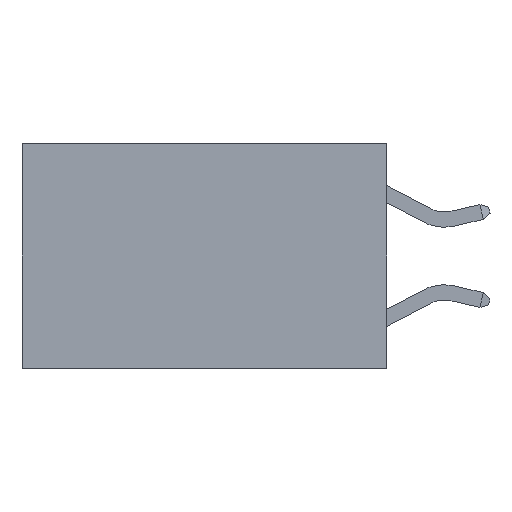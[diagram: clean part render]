
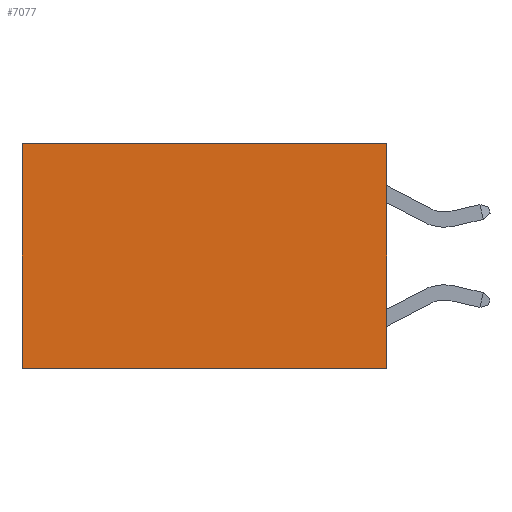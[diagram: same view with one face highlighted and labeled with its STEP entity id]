
A CAD part, left-side view. The second image highlights one B-rep face of the part: STEP entity #7077.
In plain terms, the highlighted planar face has unit normal (-1, 0, 0).
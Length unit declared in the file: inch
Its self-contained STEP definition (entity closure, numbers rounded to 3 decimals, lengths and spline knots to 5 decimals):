
#49 = DIRECTION ( 'NONE',  ( 1., 0., 0. ) ) ;
#55 = DIRECTION ( 'NONE',  ( 0., 1., 0. ) ) ;
#321 = VERTEX_POINT ( 'NONE', #4754 ) ;
#524 = VECTOR ( 'NONE', #3076, 39.37008 ) ;
#546 = DIRECTION ( 'NONE',  ( 0., 0., -1. ) ) ;
#702 = FACE_OUTER_BOUND ( 'NONE', #2381, .T. ) ;
#733 = VERTEX_POINT ( 'NONE', #5669 ) ;
#987 = VECTOR ( 'NONE', #546, 39.37008 ) ;
#1136 = VECTOR ( 'NONE', #55, 39.37008 ) ;
#2381 = EDGE_LOOP ( 'NONE', ( #4313, #6332, #2769, #6611 ) ) ;
#2558 = EDGE_CURVE ( 'NONE', #733, #8007, #2902, .T. ) ;
#2674 = CARTESIAN_POINT ( 'NONE',  ( 0.2625, 0.6, 0. ) ) ;
#2769 = ORIENTED_EDGE ( 'NONE', *, *, #6061, .F. ) ;
#2902 = LINE ( 'NONE', #8003, #524 ) ;
#3076 = DIRECTION ( 'NONE',  ( 0., 1., 0. ) ) ;
#3122 = EDGE_CURVE ( 'NONE', #8972, #8007, #4651, .T. ) ;
#3364 = EDGE_CURVE ( 'NONE', #321, #8972, #6470, .T. ) ;
#4265 = PLANE ( 'NONE',  #4604 ) ;
#4313 = ORIENTED_EDGE ( 'NONE', *, *, #3122, .T. ) ;
#4604 = AXIS2_PLACEMENT_3D ( 'NONE', #5759, #49, #6464 ) ;
#4651 = LINE ( 'NONE', #7551, #5042 ) ;
#4754 = CARTESIAN_POINT ( 'NONE',  ( 0.2625, 0., 0. ) ) ;
#4815 = CARTESIAN_POINT ( 'NONE',  ( 0.2625, 0., 0. ) ) ;
#5042 = VECTOR ( 'NONE', #6048, 39.37008 ) ;
#5669 = CARTESIAN_POINT ( 'NONE',  ( 0.2625, 0., -0.37 ) ) ;
#5759 = CARTESIAN_POINT ( 'NONE',  ( 0.2625, 0., 0. ) ) ;
#6048 = DIRECTION ( 'NONE',  ( 0., 0., -1. ) ) ;
#6061 = EDGE_CURVE ( 'NONE', #321, #733, #6131, .T. ) ;
#6131 = LINE ( 'NONE', #4815, #987 ) ;
#6332 = ORIENTED_EDGE ( 'NONE', *, *, #2558, .F. ) ;
#6343 = CARTESIAN_POINT ( 'NONE',  ( 0.2625, 0.6, -0.37 ) ) ;
#6464 = DIRECTION ( 'NONE',  ( 0., 0., -1. ) ) ;
#6470 = LINE ( 'NONE', #8429, #1136 ) ;
#6611 = ORIENTED_EDGE ( 'NONE', *, *, #3364, .T. ) ;
#7077 = ADVANCED_FACE ( 'NONE', ( #702 ), #4265, .F. ) ;
#7551 = CARTESIAN_POINT ( 'NONE',  ( 0.2625, 0.6, 0. ) ) ;
#8003 = CARTESIAN_POINT ( 'NONE',  ( 0.2625, 0., -0.37 ) ) ;
#8007 = VERTEX_POINT ( 'NONE', #6343 ) ;
#8429 = CARTESIAN_POINT ( 'NONE',  ( 0.2625, 0., 0. ) ) ;
#8972 = VERTEX_POINT ( 'NONE', #2674 ) ;
